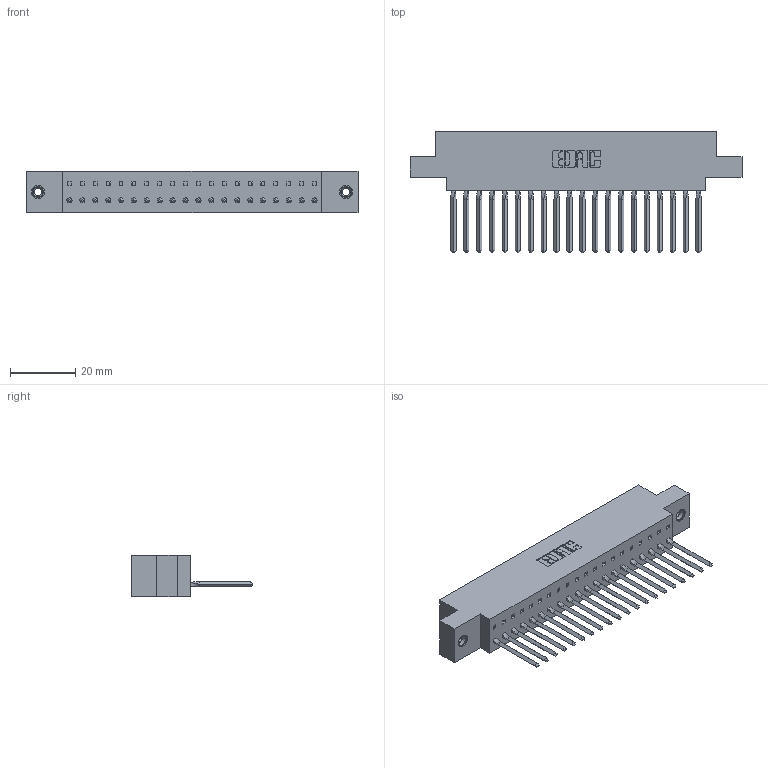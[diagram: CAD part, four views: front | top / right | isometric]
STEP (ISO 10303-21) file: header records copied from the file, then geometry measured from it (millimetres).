
FILE_DESCRIPTION (( 'STEP AP203' ), '1' );
FILE_NAME ('317-020-541-678.STEP', '2020-02-27T16:38:09', ( '' ), ( '' ), 'SwSTEP 2.0', 'SolidWorks 2016', '' );
FILE_SCHEMA (( 'CONFIG_CONTROL_DESIGN' ));
Length unit declared in the file: inch
Products named in the file (4): 317-290-002_541; 345-250-001_345-250-003-102; 317-020-541-678; 317 Part_.156 Dia - TI
Assembly tree (23 placements, depth 2):
  317-020-541-678
    317 Part_.156 Dia - TI
    317-290-002_541  x20
    345-250-001_345-250-003-102  x2
Bounding box: 101.96 x 37.34 x 12.7 mm (x, y, z)
Volume: 15850.8 mm3; surface area: 21686.3 mm2
Topology: 23 solids, 23 shells, 3202 faces, 9091 edges, 5906 vertices
Faces by surface type: plane 2570, cylinder 536, bspline 80, cone 12, torus 4
Entity records: 34073 total; most frequent: CARTESIAN_POINT 6656, ORIENTED_EDGE 5922, DIRECTION 4891, EDGE_CURVE 2961, LINE 2577, VECTOR 2577, VERTEX_POINT 1962, AXIS2_PLACEMENT_3D 1157
